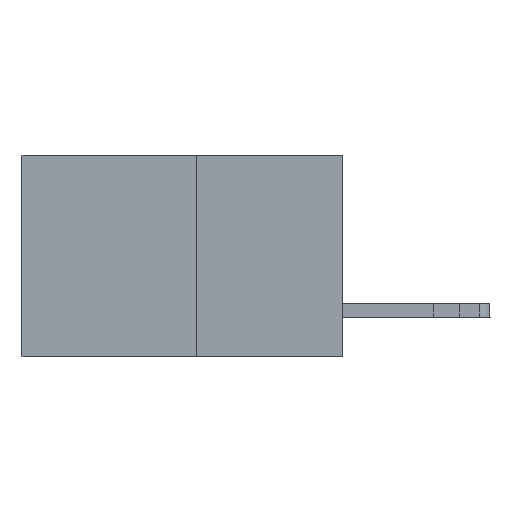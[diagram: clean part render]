
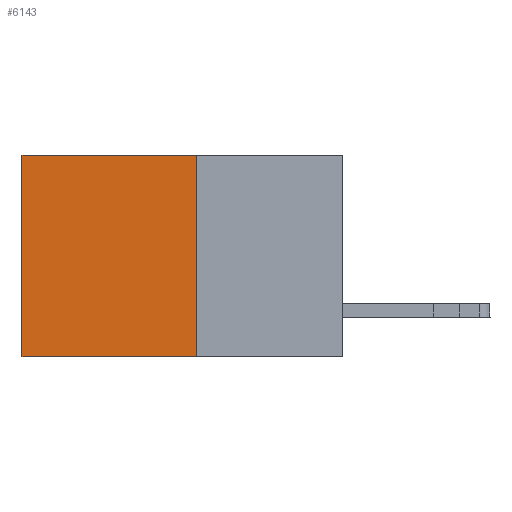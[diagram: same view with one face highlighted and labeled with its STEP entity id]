
A CAD part, left-side view. The second image highlights one B-rep face of the part: STEP entity #6143.
In plain terms, the highlighted planar face has unit normal (-1, 0, 0).
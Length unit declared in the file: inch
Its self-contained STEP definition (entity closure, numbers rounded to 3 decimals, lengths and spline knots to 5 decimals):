
#508 = ORIENTED_EDGE ( 'NONE', *, *, #12419, .F. ) ;
#1256 = LINE ( 'NONE', #5857, #5223 ) ;
#1371 = DIRECTION ( 'NONE',  ( 1., 0., 0. ) ) ;
#1481 = DIRECTION ( 'NONE',  ( 0., 1., 0. ) ) ;
#1727 = CARTESIAN_POINT ( 'NONE',  ( 0.277, 0.59, -0.37 ) ) ;
#2353 = PLANE ( 'NONE',  #5809 ) ;
#3476 = FACE_OUTER_BOUND ( 'NONE', #12600, .T. ) ;
#4735 = CARTESIAN_POINT ( 'NONE',  ( 0.277, 0.27, 0. ) ) ;
#5223 = VECTOR ( 'NONE', #12773, 39.37008 ) ;
#5809 = AXIS2_PLACEMENT_3D ( 'NONE', #11534, #1371, #13867 ) ;
#5857 = CARTESIAN_POINT ( 'NONE',  ( 0.277, 0.27, -0.37 ) ) ;
#6003 = CARTESIAN_POINT ( 'NONE',  ( 0.277, 0.27, 0. ) ) ;
#6143 = ADVANCED_FACE ( 'NONE', ( #3476 ), #2353, .F. ) ;
#6715 = CARTESIAN_POINT ( 'NONE',  ( 0.277, 0.27, -0.37 ) ) ;
#7151 = ORIENTED_EDGE ( 'NONE', *, *, #10138, .F. ) ;
#7302 = EDGE_CURVE ( 'NONE', #10201, #13132, #12010, .T. ) ;
#7499 = CARTESIAN_POINT ( 'NONE',  ( 0.277, 0.59, -0.37 ) ) ;
#7615 = VECTOR ( 'NONE', #13344, 39.37008 ) ;
#8228 = VECTOR ( 'NONE', #14351, 39.37008 ) ;
#8373 = ORIENTED_EDGE ( 'NONE', *, *, #8767, .T. ) ;
#8598 = CARTESIAN_POINT ( 'NONE',  ( 0.277, 0.27, -0.37 ) ) ;
#8752 = LINE ( 'NONE', #6715, #7615 ) ;
#8767 = EDGE_CURVE ( 'NONE', #10112, #10201, #11721, .T. ) ;
#10112 = VERTEX_POINT ( 'NONE', #6003 ) ;
#10138 = EDGE_CURVE ( 'NONE', #14418, #13132, #1256, .T. ) ;
#10201 = VERTEX_POINT ( 'NONE', #11571 ) ;
#10826 = ORIENTED_EDGE ( 'NONE', *, *, #7302, .T. ) ;
#11534 = CARTESIAN_POINT ( 'NONE',  ( 0.277, 0.27, -0.37 ) ) ;
#11571 = CARTESIAN_POINT ( 'NONE',  ( 0.277, 0.59, 0. ) ) ;
#11721 = LINE ( 'NONE', #4735, #13334 ) ;
#12010 = LINE ( 'NONE', #7499, #8228 ) ;
#12419 = EDGE_CURVE ( 'NONE', #10112, #14418, #8752, .T. ) ;
#12600 = EDGE_LOOP ( 'NONE', ( #10826, #7151, #508, #8373 ) ) ;
#12773 = DIRECTION ( 'NONE',  ( 0., 1., 0. ) ) ;
#13132 = VERTEX_POINT ( 'NONE', #1727 ) ;
#13334 = VECTOR ( 'NONE', #1481, 39.37008 ) ;
#13344 = DIRECTION ( 'NONE',  ( 0., 0., -1. ) ) ;
#13867 = DIRECTION ( 'NONE',  ( 0., 0., -1. ) ) ;
#14351 = DIRECTION ( 'NONE',  ( 0., 0., -1. ) ) ;
#14418 = VERTEX_POINT ( 'NONE', #8598 ) ;
